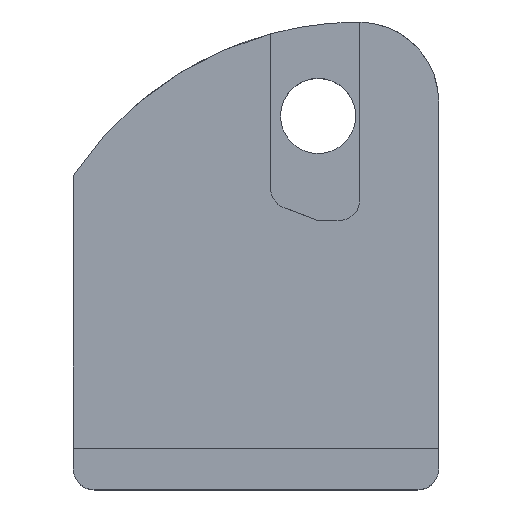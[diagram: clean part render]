
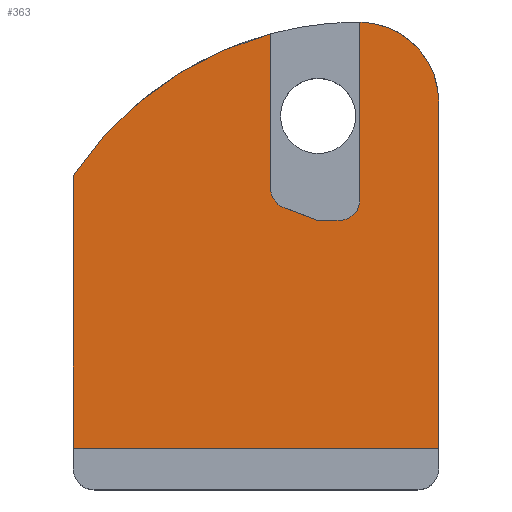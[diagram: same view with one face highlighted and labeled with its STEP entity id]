
A CAD part, top view. The second image highlights one B-rep face of the part: STEP entity #363.
In plain terms, the highlighted planar face has unit normal (0, 0, 1).
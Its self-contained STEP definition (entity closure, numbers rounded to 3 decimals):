
#18=PLANE('',#400);
#31=FACE_OUTER_BOUND('',#51,.T.);
#51=EDGE_LOOP('',(#255,#256,#257,#258,#259,#260,#261,#262,#263,#264,#265));
#75=LINE('',#561,#111);
#76=LINE('',#565,#112);
#77=LINE('',#567,#113);
#78=LINE('',#571,#114);
#79=LINE('',#575,#115);
#80=LINE('',#577,#116);
#81=LINE('',#578,#117);
#111=VECTOR('',#448,10.);
#112=VECTOR('',#451,10.);
#113=VECTOR('',#452,10.);
#114=VECTOR('',#455,10.);
#115=VECTOR('',#458,10.);
#116=VECTOR('',#459,10.);
#117=VECTOR('',#460,10.);
#146=CIRCLE('',#399,3.832);
#147=CIRCLE('',#401,1.);
#148=CIRCLE('',#402,1.);
#149=CIRCLE('',#403,16.475);
#165=VERTEX_POINT('',#554);
#166=VERTEX_POINT('',#556);
#167=VERTEX_POINT('',#560);
#168=VERTEX_POINT('',#562);
#169=VERTEX_POINT('',#564);
#170=VERTEX_POINT('',#566);
#171=VERTEX_POINT('',#568);
#172=VERTEX_POINT('',#570);
#173=VERTEX_POINT('',#572);
#174=VERTEX_POINT('',#574);
#175=VERTEX_POINT('',#576);
#200=EDGE_CURVE('',#165,#166,#146,.T.);
#202=EDGE_CURVE('',#165,#167,#75,.T.);
#203=EDGE_CURVE('',#168,#167,#147,.F.);
#204=EDGE_CURVE('',#168,#169,#76,.T.);
#205=EDGE_CURVE('',#169,#170,#77,.T.);
#206=EDGE_CURVE('',#171,#170,#148,.F.);
#207=EDGE_CURVE('',#171,#172,#78,.T.);
#208=EDGE_CURVE('',#172,#173,#149,.F.);
#209=EDGE_CURVE('',#173,#174,#79,.T.);
#210=EDGE_CURVE('',#174,#175,#80,.T.);
#211=EDGE_CURVE('',#175,#166,#81,.T.);
#255=ORIENTED_EDGE('',*,*,#200,.F.);
#256=ORIENTED_EDGE('',*,*,#202,.T.);
#257=ORIENTED_EDGE('',*,*,#203,.F.);
#258=ORIENTED_EDGE('',*,*,#204,.T.);
#259=ORIENTED_EDGE('',*,*,#205,.T.);
#260=ORIENTED_EDGE('',*,*,#206,.F.);
#261=ORIENTED_EDGE('',*,*,#207,.T.);
#262=ORIENTED_EDGE('',*,*,#208,.T.);
#263=ORIENTED_EDGE('',*,*,#209,.T.);
#264=ORIENTED_EDGE('',*,*,#210,.T.);
#265=ORIENTED_EDGE('',*,*,#211,.T.);
#363=ADVANCED_FACE('',(#31),#18,.T.);
#399=AXIS2_PLACEMENT_3D('',#557,#443,#444);
#400=AXIS2_PLACEMENT_3D('',#559,#446,#447);
#401=AXIS2_PLACEMENT_3D('',#563,#449,#450);
#402=AXIS2_PLACEMENT_3D('',#569,#453,#454);
#403=AXIS2_PLACEMENT_3D('',#573,#456,#457);
#443=DIRECTION('center_axis',(0.,0.,-1.));
#444=DIRECTION('ref_axis',(0.706,0.709,0.));
#446=DIRECTION('center_axis',(0.,0.,1.));
#447=DIRECTION('ref_axis',(1.,0.,0.));
#448=DIRECTION('',(0.,-1.,0.));
#449=DIRECTION('center_axis',(0.,0.,-1.));
#450=DIRECTION('ref_axis',(0.707,-0.707,0.));
#451=DIRECTION('',(-1.,0.,0.));
#452=DIRECTION('',(-0.935,0.354,0.));
#453=DIRECTION('center_axis',(0.,0.,-1.));
#454=DIRECTION('ref_axis',(-0.823,-0.568,0.));
#455=DIRECTION('',(0.,1.,0.));
#456=DIRECTION('center_axis',(0.,0.,-1.));
#457=DIRECTION('ref_axis',(0.,1.,0.));
#458=DIRECTION('',(0.,-1.,0.));
#459=DIRECTION('',(1.,0.,0.));
#460=DIRECTION('',(0.,1.,0.));
#554=CARTESIAN_POINT('',(13.725,22.399,3.92));
#556=CARTESIAN_POINT('',(17.5,18.568,3.92));
#557=CARTESIAN_POINT('Origin',(13.668,18.568,3.92));
#559=CARTESIAN_POINT('Origin',(8.75,10.95,3.92));
#560=CARTESIAN_POINT('',(13.725,13.9,3.92));
#561=CARTESIAN_POINT('',(13.725,11.925,3.92));
#562=CARTESIAN_POINT('',(12.725,12.9,3.92));
#563=CARTESIAN_POINT('Origin',(12.725,13.9,3.92));
#564=CARTESIAN_POINT('',(11.705,12.9,3.92));
#565=CARTESIAN_POINT('',(10.228,12.9,3.92));
#566=CARTESIAN_POINT('',(10.091,13.511,3.92));
#567=CARTESIAN_POINT('',(9.606,13.695,3.92));
#568=CARTESIAN_POINT('',(9.445,14.447,3.92));
#569=CARTESIAN_POINT('Origin',(10.445,14.447,3.92));
#570=CARTESIAN_POINT('',(9.445,21.834,3.92));
#571=CARTESIAN_POINT('',(9.445,16.133,3.92));
#572=CARTESIAN_POINT('',(0.,15.038,3.92));
#573=CARTESIAN_POINT('Origin',(13.725,5.925,3.92));
#574=CARTESIAN_POINT('',(0.,2.,3.92));
#575=CARTESIAN_POINT('',(0.,0.,3.92));
#576=CARTESIAN_POINT('',(17.5,2.,3.92));
#577=CARTESIAN_POINT('',(13.125,2.,3.92));
#578=CARTESIAN_POINT('',(17.5,18.725,3.92));
